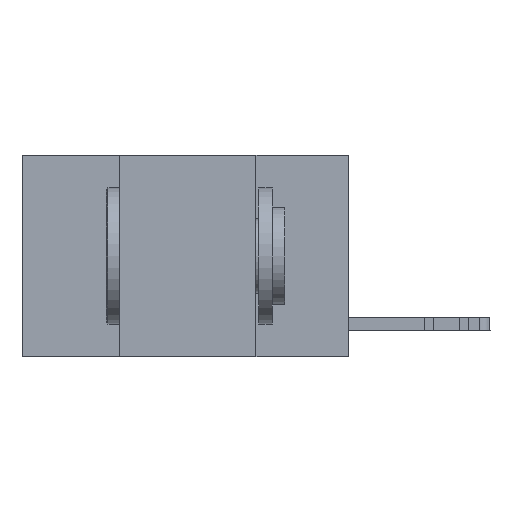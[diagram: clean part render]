
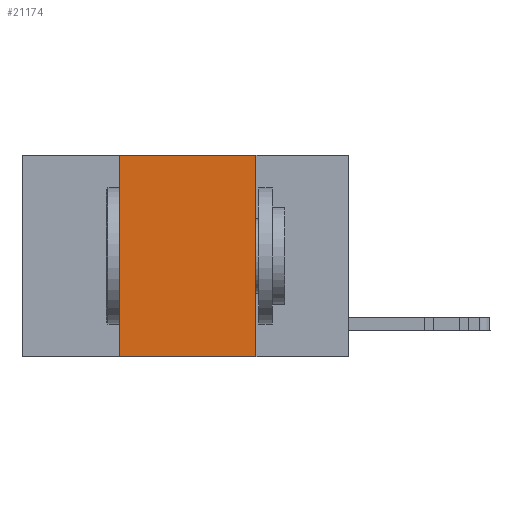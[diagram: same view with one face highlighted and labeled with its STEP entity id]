
A CAD part, left-side view. The second image highlights one B-rep face of the part: STEP entity #21174.
In plain terms, the highlighted planar face has unit normal (-1, 0, 0).
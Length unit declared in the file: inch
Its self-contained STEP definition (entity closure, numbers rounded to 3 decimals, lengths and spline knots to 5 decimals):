
#2464 = DIRECTION ( 'NONE',  ( 0., 0., 1. ) ) ;
#2644 = LINE ( 'NONE', #9773, #22787 ) ;
#3640 = VERTEX_POINT ( 'NONE', #30042 ) ;
#3752 = ORIENTED_EDGE ( 'NONE', *, *, #8329, .T. ) ;
#3936 = VECTOR ( 'NONE', #2464, 39.37008 ) ;
#5688 = FACE_OUTER_BOUND ( 'NONE', #15486, .T. ) ;
#7872 = CARTESIAN_POINT ( 'NONE',  ( 0., 0.17, -0.37 ) ) ;
#8329 = EDGE_CURVE ( 'NONE', #3640, #27125, #28584, .T. ) ;
#8646 = VECTOR ( 'NONE', #21370, 39.37008 ) ;
#8749 = VECTOR ( 'NONE', #12412, 39.37008 ) ;
#9635 = ORIENTED_EDGE ( 'NONE', *, *, #15809, .F. ) ;
#9773 = CARTESIAN_POINT ( 'NONE',  ( 0., 0.6, 0. ) ) ;
#11228 = DIRECTION ( 'NONE',  ( 0., 0., -1. ) ) ;
#12412 = DIRECTION ( 'NONE',  ( 0., -1., 0. ) ) ;
#14344 = CARTESIAN_POINT ( 'NONE',  ( 0., 0.17, 0. ) ) ;
#14816 = CARTESIAN_POINT ( 'NONE',  ( 0., 0.6, 0. ) ) ;
#15486 = EDGE_LOOP ( 'NONE', ( #9635, #27934, #20180, #3752 ) ) ;
#15492 = EDGE_CURVE ( 'NONE', #28671, #16558, #2644, .T. ) ;
#15809 = EDGE_CURVE ( 'NONE', #16558, #27125, #21517, .T. ) ;
#16057 = LINE ( 'NONE', #23367, #3936 ) ;
#16558 = VERTEX_POINT ( 'NONE', #21711 ) ;
#20180 = ORIENTED_EDGE ( 'NONE', *, *, #20641, .F. ) ;
#20641 = EDGE_CURVE ( 'NONE', #3640, #28671, #16057, .T. ) ;
#20826 = CARTESIAN_POINT ( 'NONE',  ( 0., 0.42, 0. ) ) ;
#21174 = ADVANCED_FACE ( 'NONE', ( #5688 ), #28989, .F. ) ;
#21370 = DIRECTION ( 'NONE',  ( 0., 0., -1. ) ) ;
#21517 = LINE ( 'NONE', #14344, #8646 ) ;
#21711 = CARTESIAN_POINT ( 'NONE',  ( 0., 0.17, 0. ) ) ;
#22787 = VECTOR ( 'NONE', #23554, 39.37008 ) ;
#23367 = CARTESIAN_POINT ( 'NONE',  ( 0., 0.42, 0. ) ) ;
#23554 = DIRECTION ( 'NONE',  ( 0., -1., 0. ) ) ;
#24034 = CARTESIAN_POINT ( 'NONE',  ( 0., 0.6, -0.37 ) ) ;
#27125 = VERTEX_POINT ( 'NONE', #7872 ) ;
#27440 = DIRECTION ( 'NONE',  ( 1., 0., 0. ) ) ;
#27934 = ORIENTED_EDGE ( 'NONE', *, *, #15492, .F. ) ;
#28584 = LINE ( 'NONE', #24034, #8749 ) ;
#28671 = VERTEX_POINT ( 'NONE', #20826 ) ;
#28989 = PLANE ( 'NONE',  #29267 ) ;
#29267 = AXIS2_PLACEMENT_3D ( 'NONE', #14816, #27440, #11228 ) ;
#30042 = CARTESIAN_POINT ( 'NONE',  ( 0., 0.42, -0.37 ) ) ;
